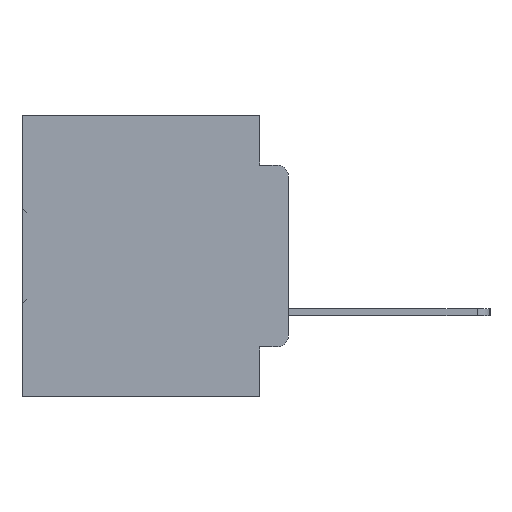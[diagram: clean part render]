
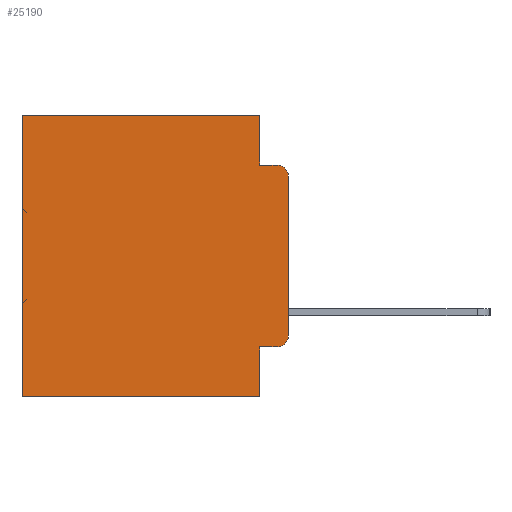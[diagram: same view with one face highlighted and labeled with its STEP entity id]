
A CAD part, left-side view. The second image highlights one B-rep face of the part: STEP entity #25190.
In plain terms, the highlighted planar face has unit normal (-1, 0, 0).
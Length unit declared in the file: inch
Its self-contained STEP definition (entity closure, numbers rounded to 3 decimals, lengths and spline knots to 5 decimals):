
#74 = CARTESIAN_POINT ( 'NONE',  ( 0.298, 0.473, -0.5 ) ) ;
#731 = EDGE_LOOP ( 'NONE', ( #26733, #13307, #6927, #15821, #1933, #12005, #33478, #14576, #29727, #9888 ) ) ;
#886 = DIRECTION ( 'NONE',  ( 0., -1., 0. ) ) ;
#1492 = CARTESIAN_POINT ( 'NONE',  ( 0.298, 0., 0. ) ) ;
#1933 = ORIENTED_EDGE ( 'NONE', *, *, #31341, .T. ) ;
#2570 = VECTOR ( 'NONE', #14085, 39.37008 ) ;
#3998 = VECTOR ( 'NONE', #14580, 39.37008 ) ;
#4189 = VERTEX_POINT ( 'NONE', #25939 ) ;
#4244 = CARTESIAN_POINT ( 'NONE',  ( 0.298, 0.02, -0.1085 ) ) ;
#4576 = LINE ( 'NONE', #33641, #18190 ) ;
#5186 = VECTOR ( 'NONE', #20771, 39.37008 ) ;
#5356 = DIRECTION ( 'NONE',  ( 0., 1., 0. ) ) ;
#5469 = VECTOR ( 'NONE', #5356, 39.37008 ) ;
#5887 = CARTESIAN_POINT ( 'NONE',  ( 0.298, 0.051, -0.0885 ) ) ;
#5969 = EDGE_CURVE ( 'NONE', #4189, #7520, #26745, .T. ) ;
#6334 = VERTEX_POINT ( 'NONE', #15003 ) ;
#6927 = ORIENTED_EDGE ( 'NONE', *, *, #28292, .F. ) ;
#6981 = AXIS2_PLACEMENT_3D ( 'NONE', #4244, #23205, #7080 ) ;
#7080 = DIRECTION ( 'NONE',  ( 0., 0., -1. ) ) ;
#7520 = VERTEX_POINT ( 'NONE', #26075 ) ;
#8646 = LINE ( 'NONE', #27790, #30126 ) ;
#9227 = VERTEX_POINT ( 'NONE', #74 ) ;
#9326 = LINE ( 'NONE', #27154, #23636 ) ;
#9888 = ORIENTED_EDGE ( 'NONE', *, *, #10282, .T. ) ;
#9992 = LINE ( 'NONE', #30173, #2570 ) ;
#10282 = EDGE_CURVE ( 'NONE', #13106, #7520, #28371, .T. ) ;
#10297 = PLANE ( 'NONE',  #20282 ) ;
#10506 = FACE_OUTER_BOUND ( 'NONE', #731, .T. ) ;
#11047 = VERTEX_POINT ( 'NONE', #26302 ) ;
#11207 = VECTOR ( 'NONE', #18048, 39.37008 ) ;
#11334 = LINE ( 'NONE', #22540, #3998 ) ;
#11706 = DIRECTION ( 'NONE',  ( 0., 0., -1. ) ) ;
#12005 = ORIENTED_EDGE ( 'NONE', *, *, #19330, .T. ) ;
#12092 = EDGE_CURVE ( 'NONE', #23131, #13106, #4576, .T. ) ;
#12160 = CARTESIAN_POINT ( 'NONE',  ( 0.298, 0.051, -0.5 ) ) ;
#12726 = CARTESIAN_POINT ( 'NONE',  ( 0.298, 0.02, -0.3915 ) ) ;
#13106 = VERTEX_POINT ( 'NONE', #13401 ) ;
#13292 = CARTESIAN_POINT ( 'NONE',  ( 0.298, 0., 0. ) ) ;
#13307 = ORIENTED_EDGE ( 'NONE', *, *, #35486, .T. ) ;
#13401 = CARTESIAN_POINT ( 'NONE',  ( 0.298, 0.02, -0.4115 ) ) ;
#14059 = CIRCLE ( 'NONE', #6981, 0.02 ) ;
#14085 = DIRECTION ( 'NONE',  ( 0., 0., -1. ) ) ;
#14576 = ORIENTED_EDGE ( 'NONE', *, *, #17508, .F. ) ;
#14580 = DIRECTION ( 'NONE',  ( 0., 0., -1. ) ) ;
#15003 = CARTESIAN_POINT ( 'NONE',  ( 0.298, 0.051, 0. ) ) ;
#15455 = DIRECTION ( 'NONE',  ( 0., 0., -1. ) ) ;
#15821 = ORIENTED_EDGE ( 'NONE', *, *, #26508, .F. ) ;
#15990 = DIRECTION ( 'NONE',  ( 0., 0., -1. ) ) ;
#16932 = VERTEX_POINT ( 'NONE', #34020 ) ;
#17508 = EDGE_CURVE ( 'NONE', #23131, #22921, #9992, .T. ) ;
#18048 = DIRECTION ( 'NONE',  ( 0., -1., 0. ) ) ;
#18190 = VECTOR ( 'NONE', #886, 39.37008 ) ;
#19023 = LINE ( 'NONE', #21556, #5469 ) ;
#19180 = DIRECTION ( 'NONE',  ( 0., 1., 0. ) ) ;
#19330 = EDGE_CURVE ( 'NONE', #16932, #9227, #8646, .T. ) ;
#20282 = AXIS2_PLACEMENT_3D ( 'NONE', #13292, #32067, #15990 ) ;
#20621 = CARTESIAN_POINT ( 'NONE',  ( 0.298, 0.051, -0.0885 ) ) ;
#20771 = DIRECTION ( 'NONE',  ( 0., 0., -1. ) ) ;
#21556 = CARTESIAN_POINT ( 'NONE',  ( 0.298, 0., -0.5 ) ) ;
#22540 = CARTESIAN_POINT ( 'NONE',  ( 0.298, 0.051, 0. ) ) ;
#22921 = VERTEX_POINT ( 'NONE', #12160 ) ;
#23131 = VERTEX_POINT ( 'NONE', #26737 ) ;
#23146 = EDGE_CURVE ( 'NONE', #22921, #9227, #19023, .T. ) ;
#23205 = DIRECTION ( 'NONE',  ( -1., 0., 0. ) ) ;
#23636 = VECTOR ( 'NONE', #19180, 39.37008 ) ;
#25190 = ADVANCED_FACE ( 'NONE', ( #10506 ), #10297, .F. ) ;
#25939 = CARTESIAN_POINT ( 'NONE',  ( 0.298, 0., -0.1085 ) ) ;
#26075 = CARTESIAN_POINT ( 'NONE',  ( 0.298, 0., -0.3915 ) ) ;
#26302 = CARTESIAN_POINT ( 'NONE',  ( 0.298, 0.02, -0.0885 ) ) ;
#26508 = EDGE_CURVE ( 'NONE', #6334, #27074, #11334, .T. ) ;
#26733 = ORIENTED_EDGE ( 'NONE', *, *, #5969, .F. ) ;
#26737 = CARTESIAN_POINT ( 'NONE',  ( 0.298, 0.051, -0.4115 ) ) ;
#26745 = LINE ( 'NONE', #1492, #5186 ) ;
#27074 = VERTEX_POINT ( 'NONE', #5887 ) ;
#27154 = CARTESIAN_POINT ( 'NONE',  ( 0.298, 0., 0. ) ) ;
#27790 = CARTESIAN_POINT ( 'NONE',  ( 0.298, 0.473, 0. ) ) ;
#28292 = EDGE_CURVE ( 'NONE', #27074, #11047, #33493, .T. ) ;
#28371 = CIRCLE ( 'NONE', #32798, 0.02 ) ;
#29727 = ORIENTED_EDGE ( 'NONE', *, *, #12092, .T. ) ;
#30126 = VECTOR ( 'NONE', #11706, 39.37008 ) ;
#30173 = CARTESIAN_POINT ( 'NONE',  ( 0.298, 0.051, 0. ) ) ;
#31341 = EDGE_CURVE ( 'NONE', #6334, #16932, #9326, .T. ) ;
#31513 = DIRECTION ( 'NONE',  ( -1., 0., 0. ) ) ;
#32067 = DIRECTION ( 'NONE',  ( 1., 0., 0. ) ) ;
#32798 = AXIS2_PLACEMENT_3D ( 'NONE', #12726, #31513, #15455 ) ;
#33478 = ORIENTED_EDGE ( 'NONE', *, *, #23146, .F. ) ;
#33493 = LINE ( 'NONE', #20621, #11207 ) ;
#33641 = CARTESIAN_POINT ( 'NONE',  ( 0.298, 0.051, -0.4115 ) ) ;
#34020 = CARTESIAN_POINT ( 'NONE',  ( 0.298, 0.473, 0. ) ) ;
#35486 = EDGE_CURVE ( 'NONE', #4189, #11047, #14059, .T. ) ;
